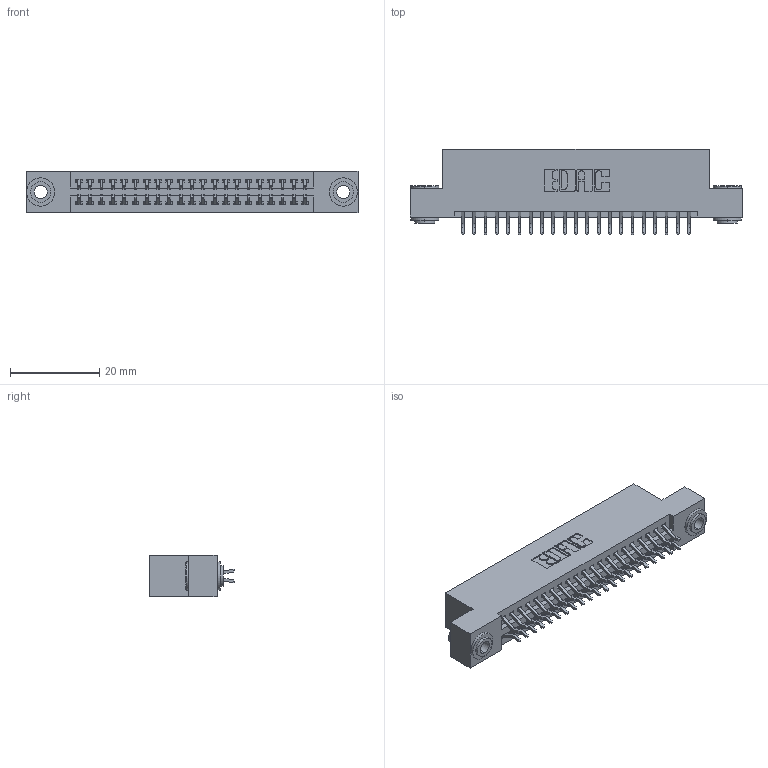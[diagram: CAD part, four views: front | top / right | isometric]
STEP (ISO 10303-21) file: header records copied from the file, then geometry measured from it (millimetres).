
FILE_DESCRIPTION (( 'STEP AP203' ), '1' );
FILE_NAME ('345-042-556-203.STEP', '2018-09-07T23:35:30', ( '' ), ( '' ), 'SwSTEP 2.0', 'SolidWorks 2016', '' );
FILE_SCHEMA (( 'CONFIG_CONTROL_DESIGN' ));
Length unit declared in the file: inch
Products named in the file (4): 345-292-001_556 Tail; 345-250-002_345-250-002-102; 345-042-556-203; 345 Part_Flush Mounting Lugs - 0.156 Dia-TH
Assembly tree (45 placements, depth 2):
  345-042-556-203
    345 Part_Flush Mounting Lugs - 0.156 Dia-TH
    345-292-001_556 Tail  x42
    345-250-002_345-250-002-102  x2
Bounding box: 74.55 x 19.24 x 9.4 mm (x, y, z)
Volume: 7064.6 mm3; surface area: 10204 mm2
Topology: 45 solids, 45 shells, 2516 faces, 7431 edges, 4894 vertices
Faces by surface type: plane 1644, cylinder 864, cone 8
Entity records: 20174 total; most frequent: CARTESIAN_POINT 3391, ORIENTED_EDGE 3306, DIRECTION 3035, EDGE_CURVE 1653, VECTOR 1405, LINE 1405, VERTEX_POINT 1098, AXIS2_PLACEMENT_3D 815
